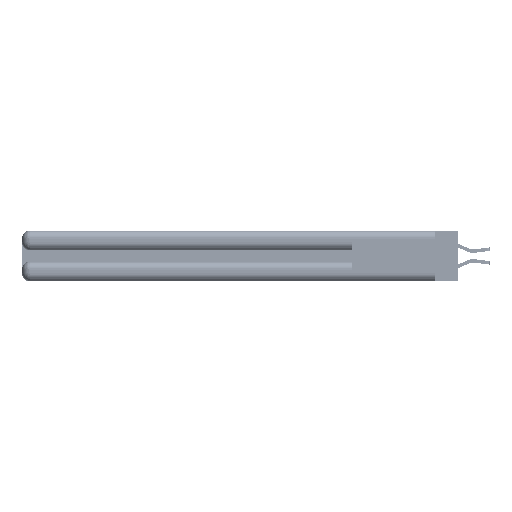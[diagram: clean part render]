
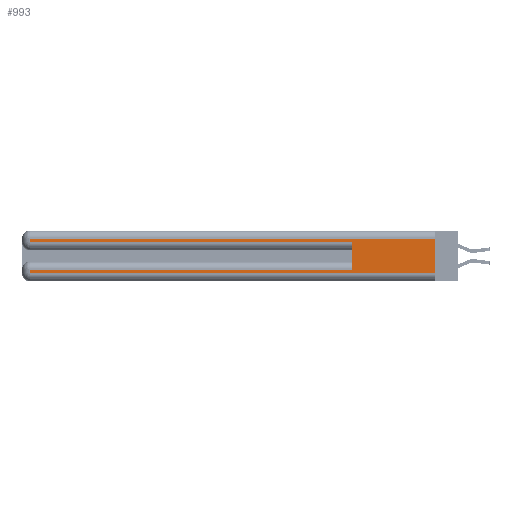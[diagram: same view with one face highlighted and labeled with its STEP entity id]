
A CAD part, left-side view. The second image highlights one B-rep face of the part: STEP entity #993.
In plain terms, the highlighted planar face has unit normal (-1, 0, 0).
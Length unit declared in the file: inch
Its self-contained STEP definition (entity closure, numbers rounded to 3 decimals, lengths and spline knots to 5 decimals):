
#91 = EDGE_CURVE ( 'NONE', #22312, #37856, #9531, .T. ) ;
#419 = EDGE_CURVE ( 'NONE', #24429, #20640, #15889, .T. ) ;
#993 = ADVANCED_FACE ( 'NONE', ( #1085 ), #33556, .F. ) ;
#1085 = FACE_OUTER_BOUND ( 'NONE', #36363, .T. ) ;
#1581 = CARTESIAN_POINT ( 'NONE',  ( 0., 0.6, 0.085 ) ) ;
#3170 = CARTESIAN_POINT ( 'NONE',  ( 0., 0., 0.285 ) ) ;
#4211 = ORIENTED_EDGE ( 'NONE', *, *, #30849, .T. ) ;
#4786 = CARTESIAN_POINT ( 'NONE',  ( 0., 2.94, 0.31 ) ) ;
#5031 = VECTOR ( 'NONE', #9969, 39.37008 ) ;
#8818 = LINE ( 'NONE', #3170, #27956 ) ;
#9017 = CARTESIAN_POINT ( 'NONE',  ( 0., 2.94, 0.06 ) ) ;
#9422 = CARTESIAN_POINT ( 'NONE',  ( 0., 0., 0.31 ) ) ;
#9474 = CARTESIAN_POINT ( 'NONE',  ( 0., 0., 0.06 ) ) ;
#9531 = LINE ( 'NONE', #24248, #41792 ) ;
#9708 = DIRECTION ( 'NONE',  ( 0., 1., 0. ) ) ;
#9969 = DIRECTION ( 'NONE',  ( 0., 0., 1. ) ) ;
#10286 = VECTOR ( 'NONE', #33813, 39.37008 ) ;
#11985 = DIRECTION ( 'NONE',  ( 0., 0., -1. ) ) ;
#12197 = VERTEX_POINT ( 'NONE', #13995 ) ;
#13871 = EDGE_CURVE ( 'NONE', #19027, #22312, #48790, .T. ) ;
#13995 = CARTESIAN_POINT ( 'NONE',  ( 0., 2.94, 0.085 ) ) ;
#14487 = EDGE_CURVE ( 'NONE', #31732, #15489, #30684, .T. ) ;
#15489 = VERTEX_POINT ( 'NONE', #38437 ) ;
#15519 = CARTESIAN_POINT ( 'NONE',  ( 0., 0.6, 0.285 ) ) ;
#15539 = DIRECTION ( 'NONE',  ( 0., -1., 0. ) ) ;
#15889 = LINE ( 'NONE', #50075, #5031 ) ;
#16250 = DIRECTION ( 'NONE',  ( 0., 0., -1. ) ) ;
#16761 = LINE ( 'NONE', #44386, #18044 ) ;
#17015 = VECTOR ( 'NONE', #20181, 39.37008 ) ;
#17645 = DIRECTION ( 'NONE',  ( 1., 0., 0. ) ) ;
#18044 = VECTOR ( 'NONE', #16250, 39.37008 ) ;
#19027 = VERTEX_POINT ( 'NONE', #9422 ) ;
#19523 = CARTESIAN_POINT ( 'NONE',  ( 0., 0., 0.085 ) ) ;
#20181 = DIRECTION ( 'NONE',  ( 0., 0., -1. ) ) ;
#20640 = VERTEX_POINT ( 'NONE', #15519 ) ;
#21876 = CARTESIAN_POINT ( 'NONE',  ( 0., 0., 0.31 ) ) ;
#21912 = CARTESIAN_POINT ( 'NONE',  ( 0., 2.94, 0.285 ) ) ;
#22312 = VERTEX_POINT ( 'NONE', #4786 ) ;
#23786 = DIRECTION ( 'NONE',  ( 0., 1., 0. ) ) ;
#24248 = CARTESIAN_POINT ( 'NONE',  ( 0., 2.94, 0.37 ) ) ;
#24429 = VERTEX_POINT ( 'NONE', #1581 ) ;
#27797 = LINE ( 'NONE', #32220, #17015 ) ;
#27956 = VECTOR ( 'NONE', #15539, 39.37008 ) ;
#29717 = CARTESIAN_POINT ( 'NONE',  ( 0., 0., 0.37 ) ) ;
#30684 = LINE ( 'NONE', #9474, #10286 ) ;
#30849 = EDGE_CURVE ( 'NONE', #12197, #31732, #27797, .T. ) ;
#31732 = VERTEX_POINT ( 'NONE', #9017 ) ;
#32220 = CARTESIAN_POINT ( 'NONE',  ( 0., 2.94, 0.37 ) ) ;
#32649 = ORIENTED_EDGE ( 'NONE', *, *, #32909, .F. ) ;
#32909 = EDGE_CURVE ( 'NONE', #19027, #15489, #16761, .T. ) ;
#33556 = PLANE ( 'NONE',  #36248 ) ;
#33813 = DIRECTION ( 'NONE',  ( 0., -1., 0. ) ) ;
#34886 = EDGE_CURVE ( 'NONE', #37856, #20640, #8818, .T. ) ;
#35368 = ORIENTED_EDGE ( 'NONE', *, *, #14487, .T. ) ;
#36248 = AXIS2_PLACEMENT_3D ( 'NONE', #29717, #17645, #45734 ) ;
#36363 = EDGE_LOOP ( 'NONE', ( #32649, #46929, #50652, #42901, #42841, #39121, #4211, #35368 ) ) ;
#37856 = VERTEX_POINT ( 'NONE', #21912 ) ;
#38249 = VECTOR ( 'NONE', #9708, 39.37008 ) ;
#38437 = CARTESIAN_POINT ( 'NONE',  ( 0., 0., 0.06 ) ) ;
#39121 = ORIENTED_EDGE ( 'NONE', *, *, #45865, .T. ) ;
#41792 = VECTOR ( 'NONE', #11985, 39.37008 ) ;
#42508 = VECTOR ( 'NONE', #23786, 39.37008 ) ;
#42841 = ORIENTED_EDGE ( 'NONE', *, *, #419, .F. ) ;
#42901 = ORIENTED_EDGE ( 'NONE', *, *, #34886, .T. ) ;
#43745 = LINE ( 'NONE', #19523, #42508 ) ;
#44386 = CARTESIAN_POINT ( 'NONE',  ( 0., 0., 0.37 ) ) ;
#45734 = DIRECTION ( 'NONE',  ( 0., 0., -1. ) ) ;
#45865 = EDGE_CURVE ( 'NONE', #24429, #12197, #43745, .T. ) ;
#46929 = ORIENTED_EDGE ( 'NONE', *, *, #13871, .T. ) ;
#48790 = LINE ( 'NONE', #21876, #38249 ) ;
#50075 = CARTESIAN_POINT ( 'NONE',  ( 0., 0.6, 0.145 ) ) ;
#50652 = ORIENTED_EDGE ( 'NONE', *, *, #91, .T. ) ;
